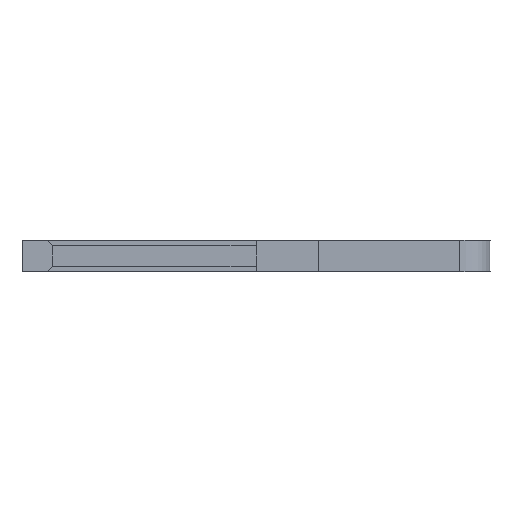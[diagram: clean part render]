
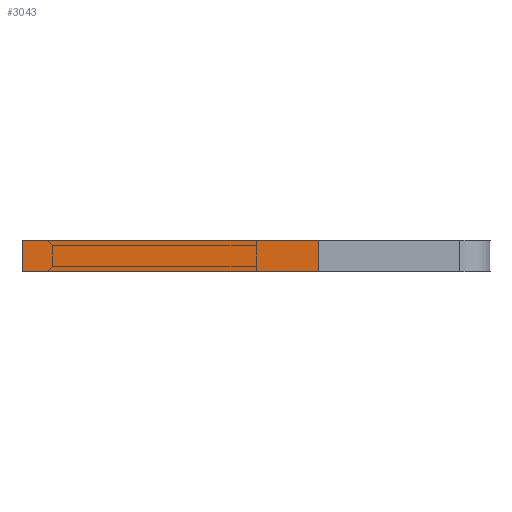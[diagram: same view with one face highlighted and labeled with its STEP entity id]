
A CAD part, left-side view. The second image highlights one B-rep face of the part: STEP entity #3043.
In plain terms, the highlighted face is planar.
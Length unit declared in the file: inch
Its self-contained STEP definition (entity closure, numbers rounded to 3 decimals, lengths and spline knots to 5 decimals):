
#16 = VERTEX_POINT ( 'NONE', #2984 ) ;
#94 = AXIS2_PLACEMENT_3D ( 'NONE', #952, #2559, #2896 ) ;
#295 = ORIENTED_EDGE ( 'NONE', *, *, #1794, .F. ) ;
#638 = EDGE_CURVE ( 'NONE', #2058, #3130, #2462, .T. ) ;
#830 = ORIENTED_EDGE ( 'NONE', *, *, #638, .F. ) ;
#952 = CARTESIAN_POINT ( 'NONE',  ( 0.01, 0.15, -0.04 ) ) ;
#1198 = CARTESIAN_POINT ( 'NONE',  ( -0.01, 0.15, -0.04 ) ) ;
#1297 = PLANE ( 'NONE',  #94 ) ;
#1466 = ORIENTED_EDGE ( 'NONE', *, *, #2371, .T. ) ;
#1468 = CARTESIAN_POINT ( 'NONE',  ( 0.01, -0.04, -0.04 ) ) ;
#1519 = LINE ( 'NONE', #3670, #2487 ) ;
#1544 = DIRECTION ( 'NONE',  ( 0., 1., 0. ) ) ;
#1715 = VECTOR ( 'NONE', #1544, 39.37008 ) ;
#1794 = EDGE_CURVE ( 'NONE', #3130, #3709, #1519, .T. ) ;
#1867 = LINE ( 'NONE', #4076, #2496 ) ;
#2058 = VERTEX_POINT ( 'NONE', #1468 ) ;
#2279 = DIRECTION ( 'NONE',  ( -1., 0., 0. ) ) ;
#2371 = EDGE_CURVE ( 'NONE', #16, #3709, #2581, .T. ) ;
#2462 = LINE ( 'NONE', #3283, #2874 ) ;
#2487 = VECTOR ( 'NONE', #3993, 39.37008 ) ;
#2496 = VECTOR ( 'NONE', #2279, 39.37008 ) ;
#2559 = DIRECTION ( 'NONE',  ( 0., 0., 1. ) ) ;
#2562 = EDGE_LOOP ( 'NONE', ( #1466, #295, #830, #3064 ) ) ;
#2581 = LINE ( 'NONE', #1198, #1715 ) ;
#2603 = CARTESIAN_POINT ( 'NONE',  ( 0.01, 0.15, -0.04 ) ) ;
#2874 = VECTOR ( 'NONE', #3582, 39.37008 ) ;
#2881 = FACE_OUTER_BOUND ( 'NONE', #2562, .T. ) ;
#2896 = DIRECTION ( 'NONE',  ( 1., 0., 0. ) ) ;
#2929 = EDGE_CURVE ( 'NONE', #2058, #16, #1867, .T. ) ;
#2984 = CARTESIAN_POINT ( 'NONE',  ( -0.01, -0.04, -0.04 ) ) ;
#3043 = ADVANCED_FACE ( 'NONE', ( #2881 ), #1297, .F. ) ;
#3064 = ORIENTED_EDGE ( 'NONE', *, *, #2929, .T. ) ;
#3130 = VERTEX_POINT ( 'NONE', #2603 ) ;
#3215 = CARTESIAN_POINT ( 'NONE',  ( -0.01, 0.15, -0.04 ) ) ;
#3283 = CARTESIAN_POINT ( 'NONE',  ( 0.01, 0.15, -0.04 ) ) ;
#3582 = DIRECTION ( 'NONE',  ( 0., 1., 0. ) ) ;
#3670 = CARTESIAN_POINT ( 'NONE',  ( 0.01, 0.15, -0.04 ) ) ;
#3709 = VERTEX_POINT ( 'NONE', #3215 ) ;
#3993 = DIRECTION ( 'NONE',  ( -1., 0., 0. ) ) ;
#4076 = CARTESIAN_POINT ( 'NONE',  ( 0.01, -0.04, -0.04 ) ) ;
